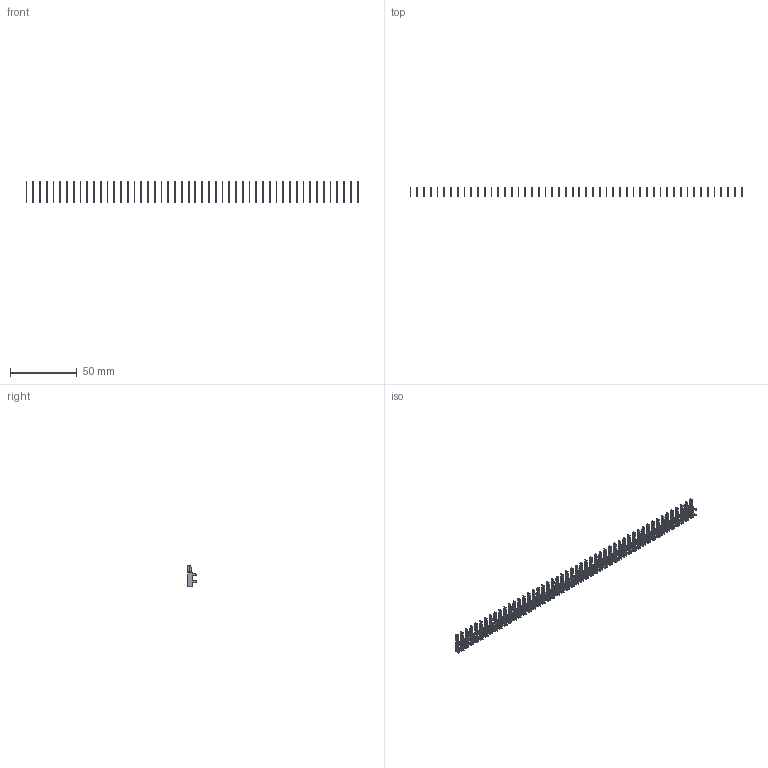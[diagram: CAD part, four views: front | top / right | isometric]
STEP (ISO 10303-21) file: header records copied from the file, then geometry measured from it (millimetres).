
FILE_DESCRIPTION (( 'STEP AP203' ), '1' );
FILE_NAME ('105-050-202-200.STEP', '2020-04-08T00:25:34', ( '' ), ( '' ), 'SwSTEP 2.0', 'SolidWorks 2016', '' );
FILE_SCHEMA (( 'CONFIG_CONTROL_DESIGN' ));
Length unit declared in the file: inch
Products named in the file (2): 100-290-001_100-290-202; 105-050-202-200
Assembly tree (50 placements, depth 2):
  105-050-202-200
    100-290-001_100-290-202  x50
Bounding box: 249.52 x 6.53 x 15.88 mm (x, y, z)
Volume: 1588.6 mm3; surface area: 7065 mm2
Topology: 50 solids, 50 shells, 1500 faces, 4200 edges, 2800 vertices
Faces by surface type: plane 1150, cylinder 350
Entity records: 2730 total; most frequent: DIRECTION 260, CARTESIAN_POINT 235, ORIENTED_EDGE 168, DATE_AND_TIME 110, COORDINATED_UNIVERSAL_TIME_OFFSET 110, CALENDAR_DATE 110, LOCAL_TIME 110, AXIS2_PLACEMENT_3D 97
